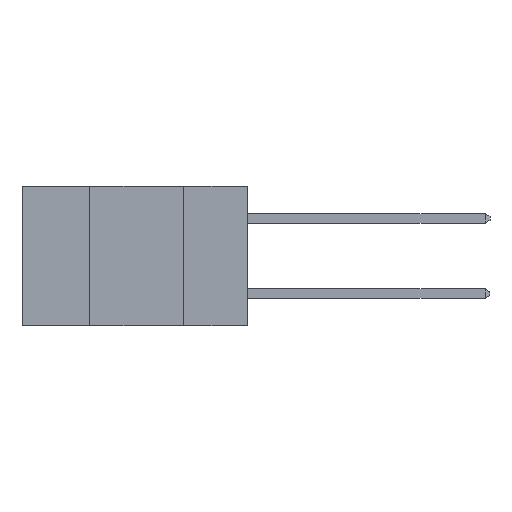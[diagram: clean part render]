
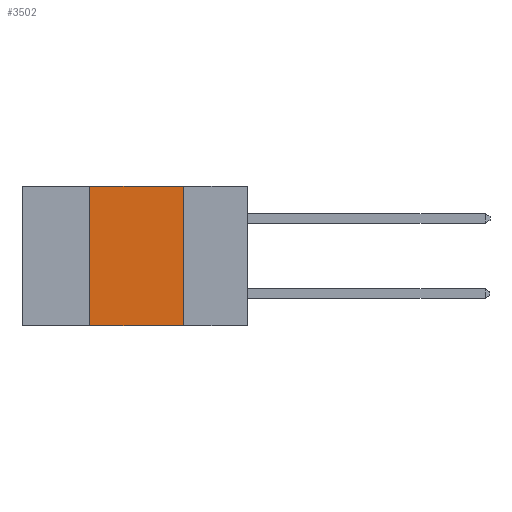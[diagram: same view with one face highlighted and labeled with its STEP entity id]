
A CAD part, left-side view. The second image highlights one B-rep face of the part: STEP entity #3502.
In plain terms, the highlighted planar face has unit normal (-1, 0, 0).
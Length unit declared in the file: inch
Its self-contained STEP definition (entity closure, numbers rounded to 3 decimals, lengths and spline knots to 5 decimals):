
#351 = EDGE_CURVE ( 'NONE', #6071, #545, #11646, .T. ) ;
#545 = VERTEX_POINT ( 'NONE', #8466 ) ;
#663 = PLANE ( 'NONE',  #9177 ) ;
#978 = CARTESIAN_POINT ( 'NONE',  ( 0., 0.42, -0.37 ) ) ;
#2323 = LINE ( 'NONE', #11505, #9573 ) ;
#3238 = DIRECTION ( 'NONE',  ( 0., 0., -1. ) ) ;
#3502 = ADVANCED_FACE ( 'NONE', ( #5436 ), #663, .F. ) ;
#3690 = ORIENTED_EDGE ( 'NONE', *, *, #4776, .F. ) ;
#3745 = DIRECTION ( 'NONE',  ( 0., -1., 0. ) ) ;
#4058 = EDGE_CURVE ( 'NONE', #10373, #9578, #4130, .T. ) ;
#4130 = LINE ( 'NONE', #6506, #11531 ) ;
#4776 = EDGE_CURVE ( 'NONE', #10373, #6071, #10067, .T. ) ;
#5307 = ORIENTED_EDGE ( 'NONE', *, *, #10194, .F. ) ;
#5436 = FACE_OUTER_BOUND ( 'NONE', #6125, .T. ) ;
#5544 = DIRECTION ( 'NONE',  ( 0., 0., 1. ) ) ;
#6071 = VERTEX_POINT ( 'NONE', #12091 ) ;
#6125 = EDGE_LOOP ( 'NONE', ( #5307, #7862, #3690, #10826 ) ) ;
#6187 = DIRECTION ( 'NONE',  ( 0., -1., 0. ) ) ;
#6506 = CARTESIAN_POINT ( 'NONE',  ( 0., 0.6, -0.37 ) ) ;
#7246 = VECTOR ( 'NONE', #3745, 39.37008 ) ;
#7342 = DIRECTION ( 'NONE',  ( 1., 0., 0. ) ) ;
#7862 = ORIENTED_EDGE ( 'NONE', *, *, #351, .F. ) ;
#8466 = CARTESIAN_POINT ( 'NONE',  ( 0., 0.17, 0. ) ) ;
#8743 = CARTESIAN_POINT ( 'NONE',  ( 0., 0.17, -0.37 ) ) ;
#9177 = AXIS2_PLACEMENT_3D ( 'NONE', #12474, #7342, #3238 ) ;
#9461 = VECTOR ( 'NONE', #5544, 39.37008 ) ;
#9573 = VECTOR ( 'NONE', #10602, 39.37008 ) ;
#9578 = VERTEX_POINT ( 'NONE', #8743 ) ;
#10067 = LINE ( 'NONE', #11667, #9461 ) ;
#10194 = EDGE_CURVE ( 'NONE', #545, #9578, #2323, .T. ) ;
#10373 = VERTEX_POINT ( 'NONE', #978 ) ;
#10602 = DIRECTION ( 'NONE',  ( 0., 0., -1. ) ) ;
#10826 = ORIENTED_EDGE ( 'NONE', *, *, #4058, .T. ) ;
#11414 = CARTESIAN_POINT ( 'NONE',  ( 0., 0.6, 0. ) ) ;
#11505 = CARTESIAN_POINT ( 'NONE',  ( 0., 0.17, 0. ) ) ;
#11531 = VECTOR ( 'NONE', #6187, 39.37008 ) ;
#11646 = LINE ( 'NONE', #11414, #7246 ) ;
#11667 = CARTESIAN_POINT ( 'NONE',  ( 0., 0.42, 0. ) ) ;
#12091 = CARTESIAN_POINT ( 'NONE',  ( 0., 0.42, 0. ) ) ;
#12474 = CARTESIAN_POINT ( 'NONE',  ( 0., 0.6, 0. ) ) ;
